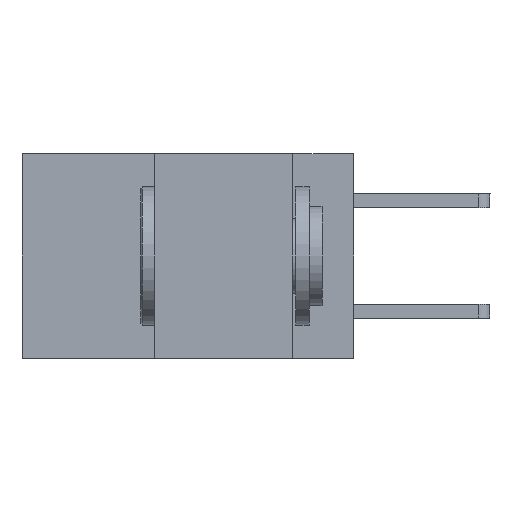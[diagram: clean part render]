
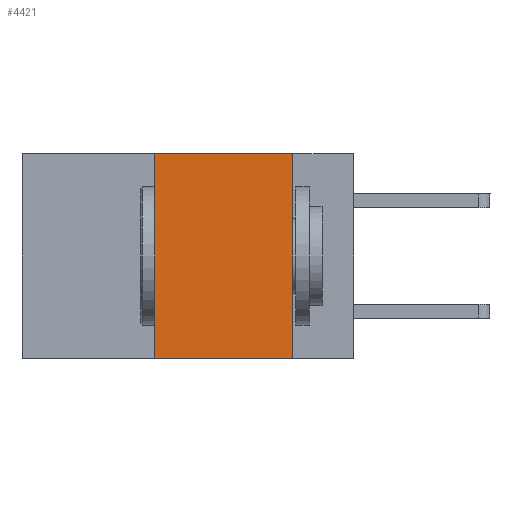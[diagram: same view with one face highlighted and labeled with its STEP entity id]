
A CAD part, left-side view. The second image highlights one B-rep face of the part: STEP entity #4421.
In plain terms, the highlighted planar face has unit normal (-1, 0, 0).
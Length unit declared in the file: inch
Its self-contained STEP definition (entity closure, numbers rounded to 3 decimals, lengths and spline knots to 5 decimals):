
#96 = VERTEX_POINT ( 'NONE', #10833 ) ;
#150 = PLANE ( 'NONE',  #10770 ) ;
#1200 = EDGE_CURVE ( 'NONE', #12169, #96, #11682, .T. ) ;
#1385 = LINE ( 'NONE', #11128, #11711 ) ;
#1980 = FACE_OUTER_BOUND ( 'NONE', #7862, .T. ) ;
#2109 = ORIENTED_EDGE ( 'NONE', *, *, #1200, .T. ) ;
#2205 = EDGE_CURVE ( 'NONE', #8208, #96, #13482, .T. ) ;
#2384 = VECTOR ( 'NONE', #9178, 39.37008 ) ;
#3017 = VECTOR ( 'NONE', #13374, 39.37008 ) ;
#3176 = CARTESIAN_POINT ( 'NONE',  ( 0., 0.6, -0.37 ) ) ;
#3216 = ORIENTED_EDGE ( 'NONE', *, *, #10425, .F. ) ;
#4311 = CARTESIAN_POINT ( 'NONE',  ( 0., 0.36, 0. ) ) ;
#4421 = ADVANCED_FACE ( 'NONE', ( #1980 ), #150, .F. ) ;
#5601 = CARTESIAN_POINT ( 'NONE',  ( 0., 0.11, 0. ) ) ;
#7479 = DIRECTION ( 'NONE',  ( 0., -1., 0. ) ) ;
#7703 = CARTESIAN_POINT ( 'NONE',  ( 0., 0.36, 0. ) ) ;
#7862 = EDGE_LOOP ( 'NONE', ( #11361, #14624, #3216, #2109 ) ) ;
#8176 = DIRECTION ( 'NONE',  ( 1., 0., 0. ) ) ;
#8208 = VERTEX_POINT ( 'NONE', #13089 ) ;
#9178 = DIRECTION ( 'NONE',  ( 0., 0., -1. ) ) ;
#9371 = CARTESIAN_POINT ( 'NONE',  ( 0., 0.6, 0. ) ) ;
#9885 = VECTOR ( 'NONE', #12030, 39.37008 ) ;
#10372 = DIRECTION ( 'NONE',  ( 0., 0., -1. ) ) ;
#10425 = EDGE_CURVE ( 'NONE', #12169, #14357, #14479, .T. ) ;
#10770 = AXIS2_PLACEMENT_3D ( 'NONE', #9371, #8176, #10372 ) ;
#10833 = CARTESIAN_POINT ( 'NONE',  ( 0., 0.11, -0.37 ) ) ;
#11128 = CARTESIAN_POINT ( 'NONE',  ( 0., 0.6, 0. ) ) ;
#11361 = ORIENTED_EDGE ( 'NONE', *, *, #2205, .F. ) ;
#11682 = LINE ( 'NONE', #3176, #9885 ) ;
#11711 = VECTOR ( 'NONE', #7479, 39.37008 ) ;
#12030 = DIRECTION ( 'NONE',  ( 0., -1., 0. ) ) ;
#12169 = VERTEX_POINT ( 'NONE', #13674 ) ;
#12584 = EDGE_CURVE ( 'NONE', #14357, #8208, #1385, .T. ) ;
#13089 = CARTESIAN_POINT ( 'NONE',  ( 0., 0.11, 0. ) ) ;
#13374 = DIRECTION ( 'NONE',  ( 0., 0., 1. ) ) ;
#13482 = LINE ( 'NONE', #5601, #2384 ) ;
#13674 = CARTESIAN_POINT ( 'NONE',  ( 0., 0.36, -0.37 ) ) ;
#14357 = VERTEX_POINT ( 'NONE', #7703 ) ;
#14479 = LINE ( 'NONE', #4311, #3017 ) ;
#14624 = ORIENTED_EDGE ( 'NONE', *, *, #12584, .F. ) ;
